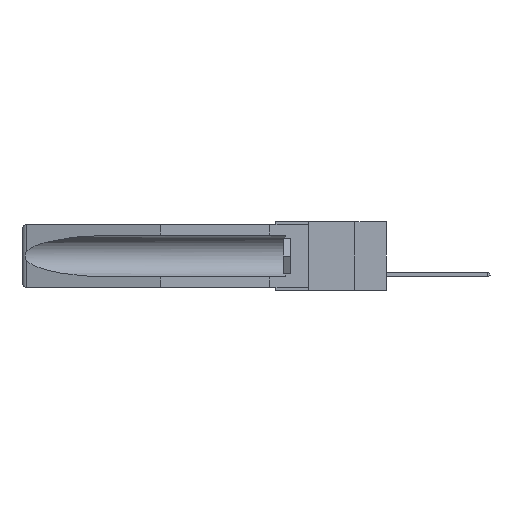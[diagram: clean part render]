
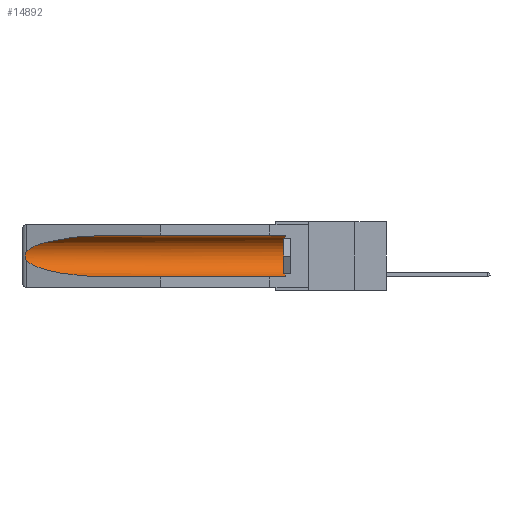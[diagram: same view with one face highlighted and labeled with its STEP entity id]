
A CAD part, left-side view. The second image highlights one B-rep face of the part: STEP entity #14892.
In plain terms, the highlighted cylindrical face has radius 2.857 mm (diameter 5.715 mm), a partial arc.
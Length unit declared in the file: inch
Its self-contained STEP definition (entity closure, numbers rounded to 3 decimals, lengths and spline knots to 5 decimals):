
#47 = ORIENTED_EDGE ( 'NONE', *, *, #25111, .F. ) ;
#1237 = CARTESIAN_POINT ( 'NONE',  ( 0.26537, 1.52718, -0.14972 ) ) ;
#1297 = CARTESIAN_POINT ( 'NONE',  ( 0.155, 1.07973, -0.284 ) ) ;
#1575 = CARTESIAN_POINT ( 'NONE',  ( 0.2673, 1.5327, -0.16383 ) ) ;
#1682 = AXIS2_PLACEMENT_3D ( 'NONE', #17447, #11209, #11501 ) ;
#2369 = EDGE_CURVE ( 'NONE', #7932, #25608, #17318, .T. ) ;
#2440 = ORIENTED_EDGE ( 'NONE', *, *, #18719, .T. ) ;
#5791 = LINE ( 'NONE', #9032, #18009 ) ;
#5849 = CARTESIAN_POINT ( 'NONE',  ( 0.26654, 1.53092, -0.15636 ) ) ;
#6151 = CARTESIAN_POINT ( 'NONE',  ( 0.2673, 1.53269, -0.17917 ) ) ;
#6902 = B_SPLINE_CURVE_WITH_KNOTS ( 'NONE', 3,
 ( #17237, #19490, #5849, #1575, #15083, #19592, #6151, #12662, #21471, #25904 ),
 .UNSPECIFIED., .F., .F.,
 ( 4, 2, 2, 2, 4 ),
 ( 0., 0.00029, 0.00058, 0.00087, 0.00117 ),
 .UNSPECIFIED. ) ;
#7118 = VERTEX_POINT ( 'NONE', #24722 ) ;
#7617 = EDGE_LOOP ( 'NONE', ( #13045, #12466, #22839, #47, #16285, #2440 ) ) ;
#7815 = LINE ( 'NONE', #27447, #28459 ) ;
#7932 = VERTEX_POINT ( 'NONE', #15807 ) ;
#8164 = EDGE_CURVE ( 'NONE', #23845, #7118, #19014, .T. ) ;
#8625 = DIRECTION ( 'NONE',  ( 0., 0., 1. ) ) ;
#9032 = CARTESIAN_POINT ( 'NONE',  ( 0.155, -0.30754, -0.059 ) ) ;
#10687 = CARTESIAN_POINT ( 'NONE',  ( 0.155, 1.07973, -0.059 ) ) ;
#10916 = EDGE_CURVE ( 'NONE', #13368, #23845, #6902, .T. ) ;
#11209 = DIRECTION ( 'NONE',  ( 0., -1., 0. ) ) ;
#11403 = FACE_OUTER_BOUND ( 'NONE', #7617, .T. ) ;
#11501 = DIRECTION ( 'NONE',  ( 0., 0., 1. ) ) ;
#11995 = CARTESIAN_POINT ( 'NONE',  ( 0.26537, 1.52718, -0.19328 ) ) ;
#12466 = ORIENTED_EDGE ( 'NONE', *, *, #10916, .T. ) ;
#12662 = CARTESIAN_POINT ( 'NONE',  ( 0.26655, 1.53094, -0.18657 ) ) ;
#12689 = CARTESIAN_POINT ( 'NONE',  ( 0.26537, 1.52718, -0.14972 ) ) ;
#12785 = CARTESIAN_POINT ( 'NONE',  ( 0.21114, 1.30732, -0.059 ) ) ;
#12995 = CARTESIAN_POINT ( 'NONE',  ( 0.155, -0.30754, -0.1715 ) ) ;
#13045 = ORIENTED_EDGE ( 'NONE', *, *, #26115, .T. ) ;
#13368 = VERTEX_POINT ( 'NONE', #1237 ) ;
#14708 = CARTESIAN_POINT ( 'NONE',  ( 0.26537, 1.52718, -0.19328 ) ) ;
#14892 = ADVANCED_FACE ( 'NONE', ( #11403 ), #17322, .F. ) ;
#15083 = CARTESIAN_POINT ( 'NONE',  ( 0.2675, 1.53308, -0.16763 ) ) ;
#15605 =( BOUNDED_CURVE ( )  B_SPLINE_CURVE ( 3, ( #20901, #12785, #26127, #12689 ),
 .UNSPECIFIED., .F., .F. ) 
 B_SPLINE_CURVE_WITH_KNOTS ( ( 4, 4 ),
 ( 4.71239, 6.08839 ),
 .UNSPECIFIED. ) 
 CURVE ( )  GEOMETRIC_REPRESENTATION_ITEM ( )  RATIONAL_B_SPLINE_CURVE ( ( 1., 0.848, 0.848, 1. ) ) 
 REPRESENTATION_ITEM ( '' )  );
#15807 = CARTESIAN_POINT ( 'NONE',  ( 0.155, 0.126, -0.284 ) ) ;
#16285 = ORIENTED_EDGE ( 'NONE', *, *, #2369, .T. ) ;
#16529 = CARTESIAN_POINT ( 'NONE',  ( 0.155, 0.126, -0.059 ) ) ;
#17237 = CARTESIAN_POINT ( 'NONE',  ( 0.26537, 1.52718, -0.14972 ) ) ;
#17318 = CIRCLE ( 'NONE', #1682, 0.1125 ) ;
#17322 = CYLINDRICAL_SURFACE ( 'NONE', #21619, 0.1125 ) ;
#17447 = CARTESIAN_POINT ( 'NONE',  ( 0.155, 0.126, -0.1715 ) ) ;
#18009 = VECTOR ( 'NONE', #27233, 39.37008 ) ;
#18719 = EDGE_CURVE ( 'NONE', #25608, #21759, #5791, .T. ) ;
#19014 =( BOUNDED_CURVE ( )  B_SPLINE_CURVE ( 3, ( #14708, #25913, #23744, #1297 ),
 .UNSPECIFIED., .F., .F. ) 
 B_SPLINE_CURVE_WITH_KNOTS ( ( 4, 4 ),
 ( 0.1948, 1.5708 ),
 .UNSPECIFIED. ) 
 CURVE ( )  GEOMETRIC_REPRESENTATION_ITEM ( )  RATIONAL_B_SPLINE_CURVE ( ( 1., 0.848, 0.848, 1. ) ) 
 REPRESENTATION_ITEM ( '' )  );
#19490 = CARTESIAN_POINT ( 'NONE',  ( 0.26597, 1.52961, -0.15275 ) ) ;
#19592 = CARTESIAN_POINT ( 'NONE',  ( 0.2675, 1.53308, -0.17534 ) ) ;
#20901 = CARTESIAN_POINT ( 'NONE',  ( 0.155, 1.07973, -0.059 ) ) ;
#21471 = CARTESIAN_POINT ( 'NONE',  ( 0.26597, 1.5296, -0.19026 ) ) ;
#21619 = AXIS2_PLACEMENT_3D ( 'NONE', #12995, #22190, #8625 ) ;
#21759 = VERTEX_POINT ( 'NONE', #10687 ) ;
#22190 = DIRECTION ( 'NONE',  ( 0., 1., 0. ) ) ;
#22839 = ORIENTED_EDGE ( 'NONE', *, *, #8164, .T. ) ;
#23744 = CARTESIAN_POINT ( 'NONE',  ( 0.21114, 1.30732, -0.284 ) ) ;
#23845 = VERTEX_POINT ( 'NONE', #11995 ) ;
#24722 = CARTESIAN_POINT ( 'NONE',  ( 0.155, 1.07973, -0.284 ) ) ;
#25111 = EDGE_CURVE ( 'NONE', #7932, #7118, #7815, .T. ) ;
#25608 = VERTEX_POINT ( 'NONE', #16529 ) ;
#25904 = CARTESIAN_POINT ( 'NONE',  ( 0.26537, 1.52718, -0.19328 ) ) ;
#25913 = CARTESIAN_POINT ( 'NONE',  ( 0.25451, 1.48313, -0.24835 ) ) ;
#25977 = DIRECTION ( 'NONE',  ( 0., 1., 0. ) ) ;
#26115 = EDGE_CURVE ( 'NONE', #21759, #13368, #15605, .T. ) ;
#26127 = CARTESIAN_POINT ( 'NONE',  ( 0.25451, 1.48313, -0.09465 ) ) ;
#27233 = DIRECTION ( 'NONE',  ( 0., 1., 0. ) ) ;
#27447 = CARTESIAN_POINT ( 'NONE',  ( 0.155, -0.30754, -0.284 ) ) ;
#28459 = VECTOR ( 'NONE', #25977, 39.37008 ) ;
